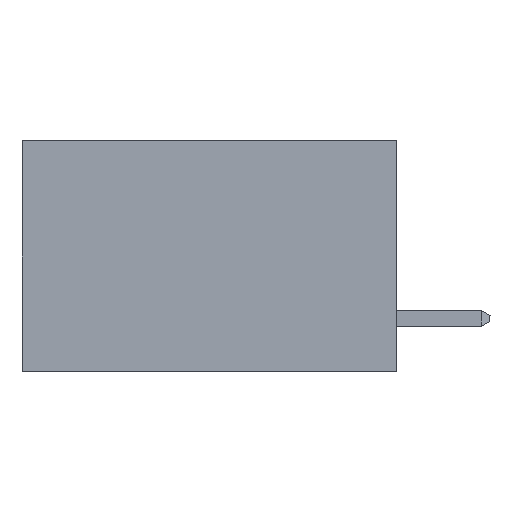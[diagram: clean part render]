
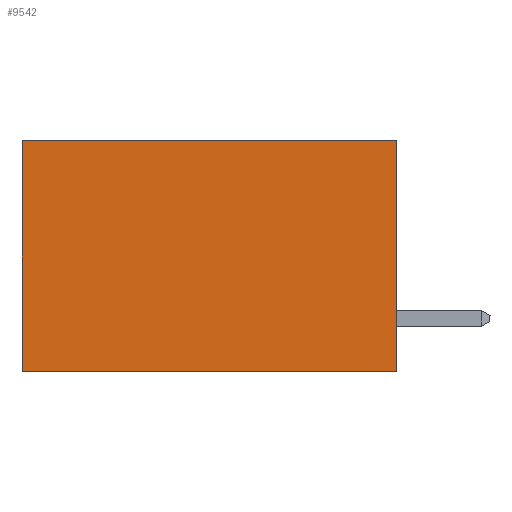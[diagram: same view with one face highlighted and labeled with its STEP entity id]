
A CAD part, left-side view. The second image highlights one B-rep face of the part: STEP entity #9542.
In plain terms, the highlighted planar face has unit normal (-1, 0, 0).
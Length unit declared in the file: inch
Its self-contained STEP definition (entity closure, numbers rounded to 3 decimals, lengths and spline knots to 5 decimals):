
#72 = EDGE_LOOP ( 'NONE', ( #8880, #10311, #9270, #11469 ) ) ;
#225 = LINE ( 'NONE', #12775, #9775 ) ;
#786 = DIRECTION ( 'NONE',  ( 0., 0., -1. ) ) ;
#889 = LINE ( 'NONE', #13714, #7117 ) ;
#1514 = CARTESIAN_POINT ( 'NONE',  ( 0.2615, 0., -0.37 ) ) ;
#2243 = CARTESIAN_POINT ( 'NONE',  ( 0.2615, 0., -0.37 ) ) ;
#3022 = CARTESIAN_POINT ( 'NONE',  ( 0.2615, 0.6, 0. ) ) ;
#3235 = CARTESIAN_POINT ( 'NONE',  ( 0.2615, 0., 0. ) ) ;
#3911 = EDGE_CURVE ( 'NONE', #7614, #9481, #889, .T. ) ;
#4201 = CARTESIAN_POINT ( 'NONE',  ( 0.2615, 0.6, -0.37 ) ) ;
#4327 = EDGE_CURVE ( 'NONE', #9481, #8620, #6834, .T. ) ;
#5493 = DIRECTION ( 'NONE',  ( 0., 1., 0. ) ) ;
#5508 = DIRECTION ( 'NONE',  ( 0., 0., -1. ) ) ;
#5887 = CARTESIAN_POINT ( 'NONE',  ( 0.2615, 0.6, -0.37 ) ) ;
#5990 = DIRECTION ( 'NONE',  ( 0., 1., 0. ) ) ;
#6834 = LINE ( 'NONE', #2243, #9256 ) ;
#7117 = VECTOR ( 'NONE', #5508, 39.37008 ) ;
#7263 = DIRECTION ( 'NONE',  ( 1., 0., 0. ) ) ;
#7425 = AXIS2_PLACEMENT_3D ( 'NONE', #8597, #7263, #10681 ) ;
#7608 = EDGE_CURVE ( 'NONE', #14403, #8620, #10264, .T. ) ;
#7614 = VERTEX_POINT ( 'NONE', #3235 ) ;
#8091 = EDGE_CURVE ( 'NONE', #7614, #14403, #225, .T. ) ;
#8597 = CARTESIAN_POINT ( 'NONE',  ( 0.2615, 0., -0.37 ) ) ;
#8620 = VERTEX_POINT ( 'NONE', #5887 ) ;
#8880 = ORIENTED_EDGE ( 'NONE', *, *, #7608, .T. ) ;
#9256 = VECTOR ( 'NONE', #5493, 39.37008 ) ;
#9270 = ORIENTED_EDGE ( 'NONE', *, *, #3911, .F. ) ;
#9481 = VERTEX_POINT ( 'NONE', #1514 ) ;
#9542 = ADVANCED_FACE ( 'NONE', ( #9562 ), #13086, .F. ) ;
#9562 = FACE_OUTER_BOUND ( 'NONE', #72, .T. ) ;
#9775 = VECTOR ( 'NONE', #5990, 39.37008 ) ;
#10264 = LINE ( 'NONE', #4201, #14313 ) ;
#10311 = ORIENTED_EDGE ( 'NONE', *, *, #4327, .F. ) ;
#10681 = DIRECTION ( 'NONE',  ( 0., 0., -1. ) ) ;
#11469 = ORIENTED_EDGE ( 'NONE', *, *, #8091, .T. ) ;
#12775 = CARTESIAN_POINT ( 'NONE',  ( 0.2615, 0., 0. ) ) ;
#13086 = PLANE ( 'NONE',  #7425 ) ;
#13714 = CARTESIAN_POINT ( 'NONE',  ( 0.2615, 0., -0.37 ) ) ;
#14313 = VECTOR ( 'NONE', #786, 39.37008 ) ;
#14403 = VERTEX_POINT ( 'NONE', #3022 ) ;
